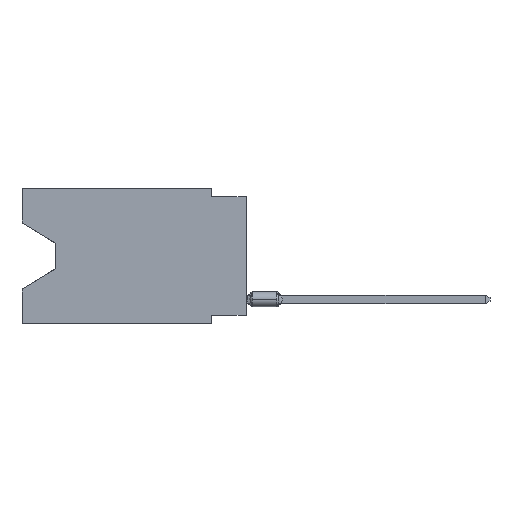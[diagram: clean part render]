
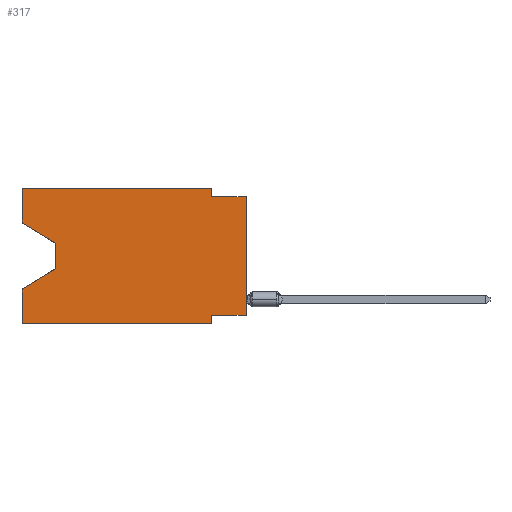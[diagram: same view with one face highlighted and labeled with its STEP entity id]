
A CAD part, left-side view. The second image highlights one B-rep face of the part: STEP entity #317.
In plain terms, the highlighted planar face has unit normal (-1, 0, 0).
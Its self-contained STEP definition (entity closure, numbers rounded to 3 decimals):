
#194 = PLANE ( 'NONE',  #10501 ) ;
#309 = EDGE_CURVE ( 'NONE', #3069, #6197, #5320, .T. ) ;
#312 = LINE ( 'NONE', #6279, #8740 ) ;
#317 = ADVANCED_FACE ( 'NONE', ( #2266 ), #194, .F. ) ;
#360 = VERTEX_POINT ( 'NONE', #9272 ) ;
#365 = CARTESIAN_POINT ( 'NONE',  ( 0., 16.383, -2.546 ) ) ;
#904 = LINE ( 'NONE', #7704, #4683 ) ;
#1120 = VERTEX_POINT ( 'NONE', #3713 ) ;
#1340 = VERTEX_POINT ( 'NONE', #5844 ) ;
#1392 = VECTOR ( 'NONE', #2303, 1000. ) ;
#1791 = LINE ( 'NONE', #5747, #5316 ) ;
#1915 = EDGE_CURVE ( 'NONE', #11807, #3069, #6022, .T. ) ;
#2022 = DIRECTION ( 'NONE',  ( 0., -0.855, -0.519 ) ) ;
#2139 = DIRECTION ( 'NONE',  ( 1., 0., 0. ) ) ;
#2266 = FACE_OUTER_BOUND ( 'NONE', #7684, .T. ) ;
#2303 = DIRECTION ( 'NONE',  ( 0., 0.855, -0.519 ) ) ;
#2438 = ORIENTED_EDGE ( 'NONE', *, *, #309, .F. ) ;
#2455 = EDGE_CURVE ( 'NONE', #360, #1340, #8082, .T. ) ;
#2517 = VECTOR ( 'NONE', #4230, 1000. ) ;
#2673 = ORIENTED_EDGE ( 'NONE', *, *, #11428, .F. ) ;
#2957 = VERTEX_POINT ( 'NONE', #9100 ) ;
#3069 = VERTEX_POINT ( 'NONE', #7842 ) ;
#3217 = CARTESIAN_POINT ( 'NONE',  ( 0., 13.97, -4.013 ) ) ;
#3359 = ORIENTED_EDGE ( 'NONE', *, *, #12481, .T. ) ;
#3496 = DIRECTION ( 'NONE',  ( 0., -1., 0. ) ) ;
#3713 = CARTESIAN_POINT ( 'NONE',  ( 0., 0., -9.271 ) ) ;
#4154 = DIRECTION ( 'NONE',  ( 0., 0., 1. ) ) ;
#4172 = ORIENTED_EDGE ( 'NONE', *, *, #1915, .F. ) ;
#4230 = DIRECTION ( 'NONE',  ( 0., 0., -1. ) ) ;
#4257 = VECTOR ( 'NONE', #5973, 1000. ) ;
#4473 = VECTOR ( 'NONE', #4154, 1000. ) ;
#4496 = VERTEX_POINT ( 'NONE', #8822 ) ;
#4683 = VECTOR ( 'NONE', #11590, 1000. ) ;
#4784 = VERTEX_POINT ( 'NONE', #3217 ) ;
#4913 = VECTOR ( 'NONE', #11929, 1000. ) ;
#5050 = ORIENTED_EDGE ( 'NONE', *, *, #12732, .T. ) ;
#5059 = DIRECTION ( 'NONE',  ( 0., 0., -1. ) ) ;
#5316 = VECTOR ( 'NONE', #9776, 1000. ) ;
#5320 = LINE ( 'NONE', #9135, #4913 ) ;
#5747 = CARTESIAN_POINT ( 'NONE',  ( 0., 0., -9.271 ) ) ;
#5844 = CARTESIAN_POINT ( 'NONE',  ( 0., 2.54, -9.906 ) ) ;
#5867 = CARTESIAN_POINT ( 'NONE',  ( 0., 2.54, 0. ) ) ;
#5973 = DIRECTION ( 'NONE',  ( 0., -1., 0. ) ) ;
#6022 = LINE ( 'NONE', #9066, #4473 ) ;
#6197 = VERTEX_POINT ( 'NONE', #5867 ) ;
#6279 = CARTESIAN_POINT ( 'NONE',  ( 0., 0., -0.635 ) ) ;
#6443 = LINE ( 'NONE', #7284, #1392 ) ;
#6522 = LINE ( 'NONE', #7362, #9877 ) ;
#6791 = EDGE_CURVE ( 'NONE', #8352, #1340, #6943, .T. ) ;
#6943 = LINE ( 'NONE', #10901, #4257 ) ;
#7236 = DIRECTION ( 'NONE',  ( 0., 0., 1. ) ) ;
#7259 = LINE ( 'NONE', #10250, #10594 ) ;
#7284 = CARTESIAN_POINT ( 'NONE',  ( 0., 13.97, -5.893 ) ) ;
#7362 = CARTESIAN_POINT ( 'NONE',  ( 0., 16.383, 0. ) ) ;
#7407 = ORIENTED_EDGE ( 'NONE', *, *, #8445, .F. ) ;
#7684 = EDGE_LOOP ( 'NONE', ( #3359, #5050, #7825, #11390, #7988, #9251, #7407, #8389, #2673, #12490, #2438, #4172 ) ) ;
#7704 = CARTESIAN_POINT ( 'NONE',  ( 0., 0., 0. ) ) ;
#7825 = ORIENTED_EDGE ( 'NONE', *, *, #8708, .T. ) ;
#7842 = CARTESIAN_POINT ( 'NONE',  ( 0., 16.383, 0. ) ) ;
#7923 = EDGE_CURVE ( 'NONE', #1120, #2957, #904, .T. ) ;
#7988 = ORIENTED_EDGE ( 'NONE', *, *, #6791, .T. ) ;
#8082 = LINE ( 'NONE', #11849, #9668 ) ;
#8204 = EDGE_CURVE ( 'NONE', #8352, #10033, #6522, .T. ) ;
#8352 = VERTEX_POINT ( 'NONE', #8659 ) ;
#8389 = ORIENTED_EDGE ( 'NONE', *, *, #7923, .T. ) ;
#8445 = EDGE_CURVE ( 'NONE', #1120, #360, #1791, .T. ) ;
#8659 = CARTESIAN_POINT ( 'NONE',  ( 0., 16.383, -9.906 ) ) ;
#8708 = EDGE_CURVE ( 'NONE', #4496, #10033, #6443, .T. ) ;
#8740 = VECTOR ( 'NONE', #3496, 1000. ) ;
#8822 = CARTESIAN_POINT ( 'NONE',  ( 0., 13.97, -5.893 ) ) ;
#9066 = CARTESIAN_POINT ( 'NONE',  ( 0., 16.383, 0. ) ) ;
#9100 = CARTESIAN_POINT ( 'NONE',  ( 0., 0., -0.635 ) ) ;
#9135 = CARTESIAN_POINT ( 'NONE',  ( 0., 16.383, 0. ) ) ;
#9142 = CARTESIAN_POINT ( 'NONE',  ( 0., 2.54, 0. ) ) ;
#9251 = ORIENTED_EDGE ( 'NONE', *, *, #2455, .F. ) ;
#9272 = CARTESIAN_POINT ( 'NONE',  ( 0., 2.54, -9.271 ) ) ;
#9369 = VECTOR ( 'NONE', #2022, 1000. ) ;
#9407 = DIRECTION ( 'NONE',  ( 0., 0., -1. ) ) ;
#9668 = VECTOR ( 'NONE', #10869, 1000. ) ;
#9776 = DIRECTION ( 'NONE',  ( 0., 1., 0. ) ) ;
#9877 = VECTOR ( 'NONE', #7236, 1000. ) ;
#9944 = LINE ( 'NONE', #10769, #9369 ) ;
#10033 = VERTEX_POINT ( 'NONE', #10915 ) ;
#10250 = CARTESIAN_POINT ( 'NONE',  ( 0., 13.97, -4.013 ) ) ;
#10501 = AXIS2_PLACEMENT_3D ( 'NONE', #11144, #2139, #5059 ) ;
#10594 = VECTOR ( 'NONE', #9407, 1000. ) ;
#10640 = EDGE_CURVE ( 'NONE', #6197, #11289, #12123, .T. ) ;
#10769 = CARTESIAN_POINT ( 'NONE',  ( 0., 16.383, -2.546 ) ) ;
#10869 = DIRECTION ( 'NONE',  ( 0., 0., -1. ) ) ;
#10901 = CARTESIAN_POINT ( 'NONE',  ( 0., 16.383, -9.906 ) ) ;
#10915 = CARTESIAN_POINT ( 'NONE',  ( 0., 16.383, -7.36 ) ) ;
#11144 = CARTESIAN_POINT ( 'NONE',  ( 0., 16.383, 0. ) ) ;
#11289 = VERTEX_POINT ( 'NONE', #11595 ) ;
#11390 = ORIENTED_EDGE ( 'NONE', *, *, #8204, .F. ) ;
#11428 = EDGE_CURVE ( 'NONE', #11289, #2957, #312, .T. ) ;
#11590 = DIRECTION ( 'NONE',  ( 0., 0., 1. ) ) ;
#11595 = CARTESIAN_POINT ( 'NONE',  ( 0., 2.54, -0.635 ) ) ;
#11807 = VERTEX_POINT ( 'NONE', #365 ) ;
#11849 = CARTESIAN_POINT ( 'NONE',  ( 0., 2.54, -9.906 ) ) ;
#11929 = DIRECTION ( 'NONE',  ( 0., -1., 0. ) ) ;
#12123 = LINE ( 'NONE', #9142, #2517 ) ;
#12481 = EDGE_CURVE ( 'NONE', #11807, #4784, #9944, .T. ) ;
#12490 = ORIENTED_EDGE ( 'NONE', *, *, #10640, .F. ) ;
#12732 = EDGE_CURVE ( 'NONE', #4784, #4496, #7259, .T. ) ;
